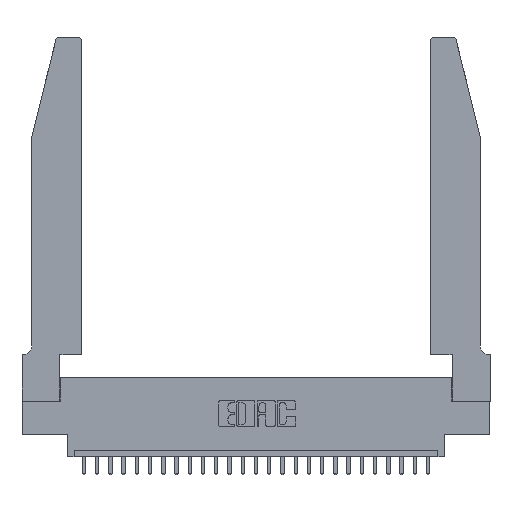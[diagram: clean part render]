
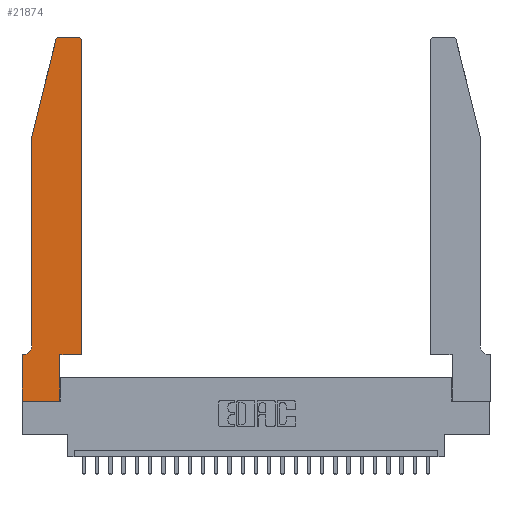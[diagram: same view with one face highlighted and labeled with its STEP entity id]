
A CAD part, top view. The second image highlights one B-rep face of the part: STEP entity #21874.
In plain terms, the highlighted planar face has unit normal (0, 0, 1).
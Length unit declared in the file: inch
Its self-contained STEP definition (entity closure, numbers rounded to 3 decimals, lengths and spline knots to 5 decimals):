
#76 = VERTEX_POINT ( 'NONE', #17714 ) ;
#729 = ORIENTED_EDGE ( 'NONE', *, *, #10113, .T. ) ;
#1651 = CIRCLE ( 'NONE', #6393, 0.03 ) ;
#2702 = ORIENTED_EDGE ( 'NONE', *, *, #24901, .T. ) ;
#3392 = DIRECTION ( 'NONE',  ( 1., 0., 0. ) ) ;
#3479 = CARTESIAN_POINT ( 'NONE',  ( 0.4505, 0.35, 0.37 ) ) ;
#3600 = EDGE_CURVE ( 'NONE', #5749, #7449, #25617, .T. ) ;
#3863 = ORIENTED_EDGE ( 'NONE', *, *, #16074, .T. ) ;
#4127 = LINE ( 'NONE', #26234, #11688 ) ;
#4634 = CARTESIAN_POINT ( 'NONE',  ( 0.284, 2.75, 0.37 ) ) ;
#4675 = ORIENTED_EDGE ( 'NONE', *, *, #17821, .T. ) ;
#4757 = CARTESIAN_POINT ( 'NONE',  ( 0.4205, 2.72, 0.37 ) ) ;
#4977 = CARTESIAN_POINT ( 'NONE',  ( 0.0755, 2., 0.37 ) ) ;
#5097 = VERTEX_POINT ( 'NONE', #16178 ) ;
#5541 = ORIENTED_EDGE ( 'NONE', *, *, #8119, .T. ) ;
#5736 = EDGE_CURVE ( 'NONE', #23727, #5749, #24175, .T. ) ;
#5749 = VERTEX_POINT ( 'NONE', #3479 ) ;
#6045 = ORIENTED_EDGE ( 'NONE', *, *, #5736, .T. ) ;
#6393 = AXIS2_PLACEMENT_3D ( 'NONE', #4757, #6858, #21625 ) ;
#6568 = DIRECTION ( 'NONE',  ( -0.239, -0.971, 0. ) ) ;
#6858 = DIRECTION ( 'NONE',  ( 0., 0., 1. ) ) ;
#7343 = CARTESIAN_POINT ( 'NONE',  ( 0.4205, 2.75, 0.37 ) ) ;
#7449 = VERTEX_POINT ( 'NONE', #21118 ) ;
#7530 = CARTESIAN_POINT ( 'NONE',  ( 0.2865, 0.35, 0.37 ) ) ;
#7720 = EDGE_LOOP ( 'NONE', ( #729, #4675, #5541, #21405, #3863, #17344, #9167, #2702, #19064, #6045, #23324, #24745 ) ) ;
#8060 = AXIS2_PLACEMENT_3D ( 'NONE', #20700, #16578, #18771 ) ;
#8119 = EDGE_CURVE ( 'NONE', #76, #20869, #11564, .T. ) ;
#8273 = CARTESIAN_POINT ( 'NONE',  ( 0.4505, 0.35, 0.37 ) ) ;
#8274 = EDGE_CURVE ( 'NONE', #20869, #5097, #16549, .T. ) ;
#8638 = DIRECTION ( 'NONE',  ( 0., -1., 0. ) ) ;
#8803 = EDGE_CURVE ( 'NONE', #7449, #19886, #1651, .T. ) ;
#9167 = ORIENTED_EDGE ( 'NONE', *, *, #21337, .T. ) ;
#9414 = DIRECTION ( 'NONE',  ( 1., 0., 0. ) ) ;
#9678 = VERTEX_POINT ( 'NONE', #15134 ) ;
#10113 = EDGE_CURVE ( 'NONE', #19886, #22053, #20696, .T. ) ;
#10265 = CARTESIAN_POINT ( 'NONE',  ( 0.2865, 0.35, 0.37 ) ) ;
#10742 = DIRECTION ( 'NONE',  ( 0., 1., 0. ) ) ;
#10798 = EDGE_CURVE ( 'NONE', #12660, #23727, #26527, .T. ) ;
#10908 = CARTESIAN_POINT ( 'NONE',  ( 0.4505, 0.35, 0.37 ) ) ;
#11564 = LINE ( 'NONE', #25453, #17885 ) ;
#11669 = VECTOR ( 'NONE', #3392, 39.37008 ) ;
#11688 = VECTOR ( 'NONE', #9414, 39.37008 ) ;
#11705 = CARTESIAN_POINT ( 'NONE',  ( 0.0755, 0.35, 0.37 ) ) ;
#12074 = DIRECTION ( 'NONE',  ( 0., 0., -1. ) ) ;
#12200 = DIRECTION ( 'NONE',  ( 0., 1., 0. ) ) ;
#12205 = PLANE ( 'NONE',  #8060 ) ;
#12660 = VERTEX_POINT ( 'NONE', #19163 ) ;
#12710 = CARTESIAN_POINT ( 'NONE',  ( 0., 0., 0.37 ) ) ;
#12820 = CARTESIAN_POINT ( 'NONE',  ( 0.2605, 2.75, 0.37 ) ) ;
#13290 = DIRECTION ( 'NONE',  ( 0., 0., 1. ) ) ;
#14472 = VECTOR ( 'NONE', #10742, 39.37008 ) ;
#14745 = VECTOR ( 'NONE', #12200, 39.37008 ) ;
#14952 = DIRECTION ( 'NONE',  ( -1., 0., 0. ) ) ;
#15134 = CARTESIAN_POINT ( 'NONE',  ( 0.0055, 0.35, 0.37 ) ) ;
#15390 = AXIS2_PLACEMENT_3D ( 'NONE', #24873, #12074, #16453 ) ;
#16074 = EDGE_CURVE ( 'NONE', #5097, #9678, #23613, .T. ) ;
#16168 = DIRECTION ( 'NONE',  ( 1., 0., 0. ) ) ;
#16178 = CARTESIAN_POINT ( 'NONE',  ( 0.0755, 0.42, 0.37 ) ) ;
#16453 = DIRECTION ( 'NONE',  ( -1., 0., 0. ) ) ;
#16549 = LINE ( 'NONE', #21864, #20479 ) ;
#16578 = DIRECTION ( 'NONE',  ( 0., 0., 1. ) ) ;
#17344 = ORIENTED_EDGE ( 'NONE', *, *, #20365, .T. ) ;
#17714 = CARTESIAN_POINT ( 'NONE',  ( 0.25487, 2.72718, 0.37 ) ) ;
#17821 = EDGE_CURVE ( 'NONE', #22053, #76, #25490, .T. ) ;
#17885 = VECTOR ( 'NONE', #6568, 39.37008 ) ;
#18728 = VECTOR ( 'NONE', #14952, 39.37008 ) ;
#18771 = DIRECTION ( 'NONE',  ( 1., 0., 0. ) ) ;
#18822 = VECTOR ( 'NONE', #26412, 39.37008 ) ;
#18868 = VERTEX_POINT ( 'NONE', #26707 ) ;
#19064 = ORIENTED_EDGE ( 'NONE', *, *, #10798, .T. ) ;
#19163 = CARTESIAN_POINT ( 'NONE',  ( 0.2865, 0., 0.37 ) ) ;
#19213 = VERTEX_POINT ( 'NONE', #23753 ) ;
#19886 = VERTEX_POINT ( 'NONE', #7343 ) ;
#20365 = EDGE_CURVE ( 'NONE', #9678, #19213, #25696, .T. ) ;
#20414 = LINE ( 'NONE', #12710, #24659 ) ;
#20479 = VECTOR ( 'NONE', #23875, 39.37008 ) ;
#20696 = LINE ( 'NONE', #12820, #18728 ) ;
#20700 = CARTESIAN_POINT ( 'NONE',  ( 0., 0.35, 0.37 ) ) ;
#20869 = VERTEX_POINT ( 'NONE', #4977 ) ;
#21118 = CARTESIAN_POINT ( 'NONE',  ( 0.4505, 2.72, 0.37 ) ) ;
#21337 = EDGE_CURVE ( 'NONE', #19213, #18868, #20414, .T. ) ;
#21405 = ORIENTED_EDGE ( 'NONE', *, *, #8274, .T. ) ;
#21467 = AXIS2_PLACEMENT_3D ( 'NONE', #25878, #13290, #16168 ) ;
#21625 = DIRECTION ( 'NONE',  ( 1., 0., 0. ) ) ;
#21864 = CARTESIAN_POINT ( 'NONE',  ( 0.0755, 2., 0.37 ) ) ;
#21874 = ADVANCED_FACE ( 'NONE', ( #26609 ), #12205, .T. ) ;
#22053 = VERTEX_POINT ( 'NONE', #4634 ) ;
#23324 = ORIENTED_EDGE ( 'NONE', *, *, #3600, .T. ) ;
#23613 = CIRCLE ( 'NONE', #15390, 0.07 ) ;
#23727 = VERTEX_POINT ( 'NONE', #7530 ) ;
#23753 = CARTESIAN_POINT ( 'NONE',  ( 0., 0.35, 0.37 ) ) ;
#23875 = DIRECTION ( 'NONE',  ( 0., -1., 0. ) ) ;
#24175 = LINE ( 'NONE', #8273, #11669 ) ;
#24659 = VECTOR ( 'NONE', #8638, 39.37008 ) ;
#24745 = ORIENTED_EDGE ( 'NONE', *, *, #8803, .T. ) ;
#24873 = CARTESIAN_POINT ( 'NONE',  ( 0.0055, 0.42, 0.37 ) ) ;
#24901 = EDGE_CURVE ( 'NONE', #18868, #12660, #4127, .T. ) ;
#25453 = CARTESIAN_POINT ( 'NONE',  ( 0.0755, 2., 0.37 ) ) ;
#25490 = CIRCLE ( 'NONE', #21467, 0.03 ) ;
#25617 = LINE ( 'NONE', #10908, #14472 ) ;
#25696 = LINE ( 'NONE', #11705, #18822 ) ;
#25878 = CARTESIAN_POINT ( 'NONE',  ( 0.284, 2.72, 0.37 ) ) ;
#26234 = CARTESIAN_POINT ( 'NONE',  ( 0., 0., 0.37 ) ) ;
#26412 = DIRECTION ( 'NONE',  ( -1., 0., 0. ) ) ;
#26527 = LINE ( 'NONE', #10265, #14745 ) ;
#26609 = FACE_OUTER_BOUND ( 'NONE', #7720, .T. ) ;
#26707 = CARTESIAN_POINT ( 'NONE',  ( 0., 0., 0.37 ) ) ;
